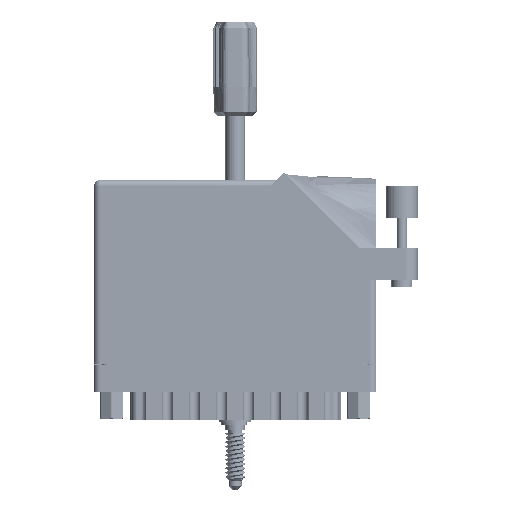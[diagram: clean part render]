
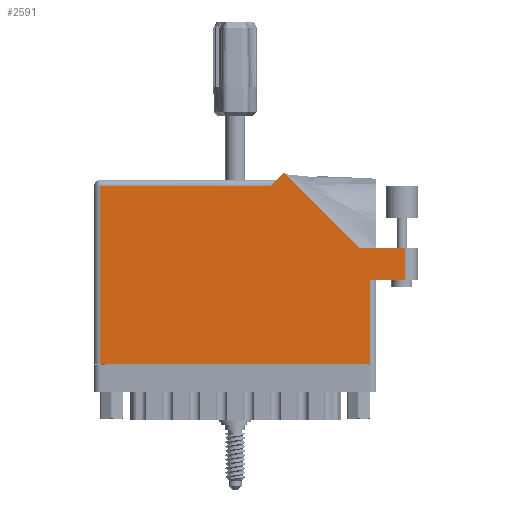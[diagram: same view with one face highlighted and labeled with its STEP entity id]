
A CAD part, front view. The second image highlights one B-rep face of the part: STEP entity #2591.
In plain terms, the highlighted face is planar.
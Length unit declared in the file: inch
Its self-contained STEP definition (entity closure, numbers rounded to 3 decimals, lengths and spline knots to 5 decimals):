
#2446 = VECTOR ( 'NONE', #82984, 39.37008 ) ;
#2591 = ADVANCED_FACE ( 'NONE', ( #59459 ), #92438, .F. ) ;
#3036 = ORIENTED_EDGE ( 'NONE', *, *, #85206, .T. ) ;
#4869 = LINE ( 'NONE', #44234, #2446 ) ;
#6574 = VERTEX_POINT ( 'NONE', #51982 ) ;
#7043 = DIRECTION ( 'NONE',  ( -1., 0., 0. ) ) ;
#10679 = DIRECTION ( 'NONE',  ( 1., 0., 0. ) ) ;
#11030 = VERTEX_POINT ( 'NONE', #39488 ) ;
#13962 = CARTESIAN_POINT ( 'NONE',  ( 1.82871, 1.84571, 0. ) ) ;
#16263 = VERTEX_POINT ( 'NONE', #75388 ) ;
#16580 = VERTEX_POINT ( 'NONE', #18502 ) ;
#16646 = DIRECTION ( 'NONE',  ( 0., 0., -1. ) ) ;
#17267 = CARTESIAN_POINT ( 'NONE',  ( 2.993, 1.122, 0. ) ) ;
#18502 = CARTESIAN_POINT ( 'NONE',  ( 0.062, 0., 0. ) ) ;
#21911 = VERTEX_POINT ( 'NONE', #75466 ) ;
#22107 = CARTESIAN_POINT ( 'NONE',  ( 1.758, 1.775, 0. ) ) ;
#22562 = LINE ( 'NONE', #86528, #83537 ) ;
#23303 = CARTESIAN_POINT ( 'NONE',  ( 0., 1.775, 0. ) ) ;
#24504 = EDGE_CURVE ( 'NONE', #37457, #16263, #27030, .T. ) ;
#25715 = CARTESIAN_POINT ( 'NONE',  ( 3.118, 1.122, 0. ) ) ;
#27030 = LINE ( 'NONE', #25715, #74867 ) ;
#30110 = LINE ( 'NONE', #87482, #82668 ) ;
#32989 = EDGE_CURVE ( 'NONE', #50025, #6574, #30110, .T. ) ;
#33278 = VERTEX_POINT ( 'NONE', #13962 ) ;
#34621 = ORIENTED_EDGE ( 'NONE', *, *, #32989, .T. ) ;
#36743 = CARTESIAN_POINT ( 'NONE',  ( 0., 1.713, 0. ) ) ;
#37457 = VERTEX_POINT ( 'NONE', #17267 ) ;
#38410 = DIRECTION ( 'NONE',  ( -0.707, 0.707, 0. ) ) ;
#39372 = CARTESIAN_POINT ( 'NONE',  ( 2.55242, 1.122, 0. ) ) ;
#39488 = CARTESIAN_POINT ( 'NONE',  ( 2.656, 0., 0. ) ) ;
#41221 = CARTESIAN_POINT ( 'NONE',  ( 2.656, 0.815, 0. ) ) ;
#43286 = CARTESIAN_POINT ( 'NONE',  ( 2.656, 0.815, 0. ) ) ;
#44234 = CARTESIAN_POINT ( 'NONE',  ( 0., 0., 0. ) ) ;
#44361 = LINE ( 'NONE', #39372, #80216 ) ;
#44484 = CARTESIAN_POINT ( 'NONE',  ( 2.993, 1.122, 0. ) ) ;
#49112 = EDGE_CURVE ( 'NONE', #16263, #33278, #44361, .T. ) ;
#50025 = VERTEX_POINT ( 'NONE', #41221 ) ;
#51824 = EDGE_LOOP ( 'NONE', ( #34621, #72634, #55507, #93363, #53198, #55557, #3036, #70086, #85547 ) ) ;
#51982 = CARTESIAN_POINT ( 'NONE',  ( 2.993, 0.815, 0. ) ) ;
#53198 = ORIENTED_EDGE ( 'NONE', *, *, #95419, .T. ) ;
#53627 = EDGE_CURVE ( 'NONE', #11030, #50025, #65742, .T. ) ;
#55507 = ORIENTED_EDGE ( 'NONE', *, *, #24504, .T. ) ;
#55557 = ORIENTED_EDGE ( 'NONE', *, *, #88593, .T. ) ;
#56183 = DIRECTION ( 'NONE',  ( 0., -1., 0. ) ) ;
#59459 = FACE_OUTER_BOUND ( 'NONE', #51824, .T. ) ;
#60191 = CARTESIAN_POINT ( 'NONE',  ( 0.062, 1.713, 0. ) ) ;
#60666 = LINE ( 'NONE', #22107, #98876 ) ;
#61015 = VECTOR ( 'NONE', #89956, 39.37008 ) ;
#61976 = EDGE_CURVE ( 'NONE', #6574, #37457, #93286, .T. ) ;
#65742 = LINE ( 'NONE', #43286, #83652 ) ;
#66353 = DIRECTION ( 'NONE',  ( 0., 1., 0. ) ) ;
#70086 = ORIENTED_EDGE ( 'NONE', *, *, #70198, .T. ) ;
#70198 = EDGE_CURVE ( 'NONE', #16580, #11030, #4869, .T. ) ;
#72634 = ORIENTED_EDGE ( 'NONE', *, *, #61976, .T. ) ;
#74807 = VERTEX_POINT ( 'NONE', #60191 ) ;
#74867 = VECTOR ( 'NONE', #78520, 39.37008 ) ;
#75388 = CARTESIAN_POINT ( 'NONE',  ( 2.55242, 1.122, 0. ) ) ;
#75466 = CARTESIAN_POINT ( 'NONE',  ( 1.696, 1.713, 0. ) ) ;
#78378 = VECTOR ( 'NONE', #7043, 39.37008 ) ;
#78520 = DIRECTION ( 'NONE',  ( -1., 0., 0. ) ) ;
#80216 = VECTOR ( 'NONE', #38410, 39.37008 ) ;
#82668 = VECTOR ( 'NONE', #10679, 39.37008 ) ;
#82984 = DIRECTION ( 'NONE',  ( 1., 0., 0. ) ) ;
#83248 = DIRECTION ( 'NONE',  ( -0.707, -0.707, 0. ) ) ;
#83537 = VECTOR ( 'NONE', #56183, 39.37008 ) ;
#83652 = VECTOR ( 'NONE', #66353, 39.37008 ) ;
#85206 = EDGE_CURVE ( 'NONE', #74807, #16580, #22562, .T. ) ;
#85547 = ORIENTED_EDGE ( 'NONE', *, *, #53627, .T. ) ;
#86528 = CARTESIAN_POINT ( 'NONE',  ( 0.062, 0., 0. ) ) ;
#87482 = CARTESIAN_POINT ( 'NONE',  ( 2.718, 0.815, 0. ) ) ;
#88593 = EDGE_CURVE ( 'NONE', #21911, #74807, #98682, .T. ) ;
#89956 = DIRECTION ( 'NONE',  ( 0., 1., 0. ) ) ;
#92438 = PLANE ( 'NONE',  #93443 ) ;
#93077 = DIRECTION ( 'NONE',  ( -1., 0., 0. ) ) ;
#93286 = LINE ( 'NONE', #44484, #61015 ) ;
#93363 = ORIENTED_EDGE ( 'NONE', *, *, #49112, .T. ) ;
#93443 = AXIS2_PLACEMENT_3D ( 'NONE', #23303, #16646, #93077 ) ;
#95419 = EDGE_CURVE ( 'NONE', #33278, #21911, #60666, .T. ) ;
#98682 = LINE ( 'NONE', #36743, #78378 ) ;
#98876 = VECTOR ( 'NONE', #83248, 39.37008 ) ;
